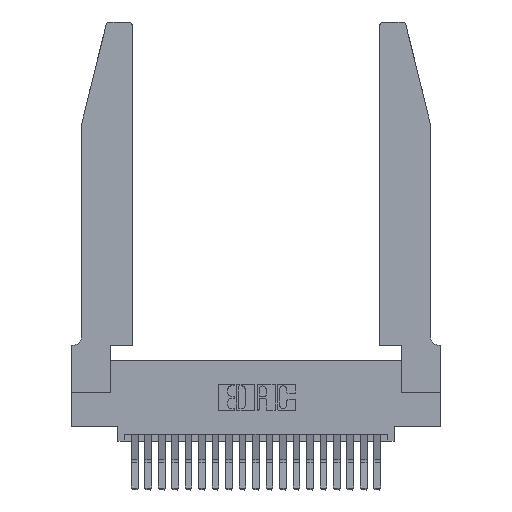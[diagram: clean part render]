
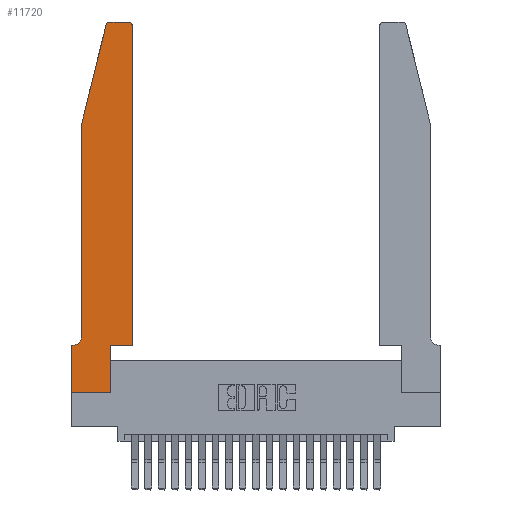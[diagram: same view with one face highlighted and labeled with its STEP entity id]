
A CAD part, top view. The second image highlights one B-rep face of the part: STEP entity #11720.
In plain terms, the highlighted planar face has unit normal (0, 0, 1).
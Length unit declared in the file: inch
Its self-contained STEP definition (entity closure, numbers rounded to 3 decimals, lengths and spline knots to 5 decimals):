
#58 = EDGE_CURVE ( 'NONE', #17497, #2567, #5552, .T. ) ;
#1557 = VECTOR ( 'NONE', #11634, 39.37008 ) ;
#1785 = CARTESIAN_POINT ( 'NONE',  ( 0.284, 2.72, 0.37 ) ) ;
#2291 = ORIENTED_EDGE ( 'NONE', *, *, #8725, .T. ) ;
#2340 = DIRECTION ( 'NONE',  ( 0., -1., 0. ) ) ;
#2380 = CARTESIAN_POINT ( 'NONE',  ( 0.0755, 0.35, 0.37 ) ) ;
#2567 = VERTEX_POINT ( 'NONE', #13069 ) ;
#2730 = VECTOR ( 'NONE', #4189, 39.37008 ) ;
#2981 = VECTOR ( 'NONE', #12494, 39.37008 ) ;
#3299 = ORIENTED_EDGE ( 'NONE', *, *, #21395, .T. ) ;
#3468 = CARTESIAN_POINT ( 'NONE',  ( 0., 0., 0.37 ) ) ;
#3584 = DIRECTION ( 'NONE',  ( 1., 0., 0. ) ) ;
#4167 = CARTESIAN_POINT ( 'NONE',  ( 0.0755, 2., 0.37 ) ) ;
#4189 = DIRECTION ( 'NONE',  ( -1., 0., 0. ) ) ;
#4584 = ORIENTED_EDGE ( 'NONE', *, *, #20979, .T. ) ;
#4935 = ORIENTED_EDGE ( 'NONE', *, *, #19337, .T. ) ;
#5075 = VERTEX_POINT ( 'NONE', #19830 ) ;
#5257 = CARTESIAN_POINT ( 'NONE',  ( 0.2865, 0., 0.37 ) ) ;
#5339 = VERTEX_POINT ( 'NONE', #6552 ) ;
#5552 = LINE ( 'NONE', #21152, #9830 ) ;
#5629 = CARTESIAN_POINT ( 'NONE',  ( 0., 0., 0.37 ) ) ;
#5875 = ORIENTED_EDGE ( 'NONE', *, *, #17522, .T. ) ;
#6082 = DIRECTION ( 'NONE',  ( 0., 0., -1. ) ) ;
#6132 = ORIENTED_EDGE ( 'NONE', *, *, #7724, .T. ) ;
#6315 = DIRECTION ( 'NONE',  ( -1., 0., 0. ) ) ;
#6552 = CARTESIAN_POINT ( 'NONE',  ( 0.4205, 2.75, 0.37 ) ) ;
#6965 = VERTEX_POINT ( 'NONE', #11075 ) ;
#7152 = DIRECTION ( 'NONE',  ( 0., 0., 1. ) ) ;
#7724 = EDGE_CURVE ( 'NONE', #5075, #22761, #13588, .T. ) ;
#8382 = CARTESIAN_POINT ( 'NONE',  ( 0.284, 2.75, 0.37 ) ) ;
#8436 = CARTESIAN_POINT ( 'NONE',  ( 0.4505, 0.35, 0.37 ) ) ;
#8725 = EDGE_CURVE ( 'NONE', #19949, #5339, #14077, .T. ) ;
#8833 = VECTOR ( 'NONE', #2340, 39.37008 ) ;
#8927 = LINE ( 'NONE', #15577, #14209 ) ;
#9027 = CARTESIAN_POINT ( 'NONE',  ( 0.0055, 0.35, 0.37 ) ) ;
#9386 = VECTOR ( 'NONE', #10244, 39.37008 ) ;
#9554 = CARTESIAN_POINT ( 'NONE',  ( 0.0755, 2., 0.37 ) ) ;
#9830 = VECTOR ( 'NONE', #10732, 39.37008 ) ;
#10030 = ORIENTED_EDGE ( 'NONE', *, *, #19240, .T. ) ;
#10244 = DIRECTION ( 'NONE',  ( 0., 1., 0. ) ) ;
#10634 = AXIS2_PLACEMENT_3D ( 'NONE', #16817, #6082, #18562 ) ;
#10695 = CIRCLE ( 'NONE', #16683, 0.03 ) ;
#10732 = DIRECTION ( 'NONE',  ( 0., 1., 0. ) ) ;
#11075 = CARTESIAN_POINT ( 'NONE',  ( 0.4505, 0.35, 0.37 ) ) ;
#11154 = VERTEX_POINT ( 'NONE', #5629 ) ;
#11178 = LINE ( 'NONE', #16906, #1557 ) ;
#11228 = DIRECTION ( 'NONE',  ( 1., 0., 0. ) ) ;
#11344 = EDGE_LOOP ( 'NONE', ( #19881, #5875, #3299, #6132, #4584, #16481, #21913, #4935, #15872, #10030, #12206, #2291 ) ) ;
#11634 = DIRECTION ( 'NONE',  ( 1., 0., 0. ) ) ;
#11720 = ADVANCED_FACE ( 'NONE', ( #22411 ), #16497, .T. ) ;
#12206 = ORIENTED_EDGE ( 'NONE', *, *, #22265, .T. ) ;
#12328 = LINE ( 'NONE', #2380, #2730 ) ;
#12494 = DIRECTION ( 'NONE',  ( 0., -1., 0. ) ) ;
#12583 = LINE ( 'NONE', #3468, #2981 ) ;
#12665 = LINE ( 'NONE', #20442, #16833 ) ;
#13056 = VECTOR ( 'NONE', #21952, 39.37008 ) ;
#13069 = CARTESIAN_POINT ( 'NONE',  ( 0.2865, 0.35, 0.37 ) ) ;
#13264 = CARTESIAN_POINT ( 'NONE',  ( 0.25487, 2.72718, 0.37 ) ) ;
#13588 = LINE ( 'NONE', #9554, #8833 ) ;
#14077 = CIRCLE ( 'NONE', #21797, 0.03 ) ;
#14111 = LINE ( 'NONE', #8436, #9386 ) ;
#14209 = VECTOR ( 'NONE', #17148, 39.37008 ) ;
#14366 = DIRECTION ( 'NONE',  ( 0., 0., 1. ) ) ;
#14715 = CARTESIAN_POINT ( 'NONE',  ( 0., 0.35, 0.37 ) ) ;
#15268 = CARTESIAN_POINT ( 'NONE',  ( 0.0755, 0.42, 0.37 ) ) ;
#15559 = AXIS2_PLACEMENT_3D ( 'NONE', #14715, #21748, #11228 ) ;
#15577 = CARTESIAN_POINT ( 'NONE',  ( 0., 0., 0.37 ) ) ;
#15872 = ORIENTED_EDGE ( 'NONE', *, *, #58, .T. ) ;
#16481 = ORIENTED_EDGE ( 'NONE', *, *, #18370, .T. ) ;
#16497 = PLANE ( 'NONE',  #15559 ) ;
#16677 = CIRCLE ( 'NONE', #10634, 0.07 ) ;
#16683 = AXIS2_PLACEMENT_3D ( 'NONE', #1785, #14366, #3584 ) ;
#16817 = CARTESIAN_POINT ( 'NONE',  ( 0.0055, 0.42, 0.37 ) ) ;
#16833 = VECTOR ( 'NONE', #6315, 39.37008 ) ;
#16885 = VERTEX_POINT ( 'NONE', #9027 ) ;
#16906 = CARTESIAN_POINT ( 'NONE',  ( 0.4505, 0.35, 0.37 ) ) ;
#17148 = DIRECTION ( 'NONE',  ( 1., 0., 0. ) ) ;
#17203 = EDGE_CURVE ( 'NONE', #5339, #21588, #12665, .T. ) ;
#17497 = VERTEX_POINT ( 'NONE', #5257 ) ;
#17522 = EDGE_CURVE ( 'NONE', #21588, #19210, #10695, .T. ) ;
#17816 = CARTESIAN_POINT ( 'NONE',  ( 0.4205, 2.72, 0.37 ) ) ;
#18370 = EDGE_CURVE ( 'NONE', #16885, #21898, #12328, .T. ) ;
#18562 = DIRECTION ( 'NONE',  ( -1., 0., 0. ) ) ;
#18920 = CARTESIAN_POINT ( 'NONE',  ( 0.4505, 2.72, 0.37 ) ) ;
#18947 = EDGE_CURVE ( 'NONE', #21898, #11154, #12583, .T. ) ;
#19210 = VERTEX_POINT ( 'NONE', #13264 ) ;
#19240 = EDGE_CURVE ( 'NONE', #2567, #6965, #11178, .T. ) ;
#19337 = EDGE_CURVE ( 'NONE', #11154, #17497, #8927, .T. ) ;
#19569 = DIRECTION ( 'NONE',  ( 1., 0., 0. ) ) ;
#19830 = CARTESIAN_POINT ( 'NONE',  ( 0.0755, 2., 0.37 ) ) ;
#19881 = ORIENTED_EDGE ( 'NONE', *, *, #17203, .T. ) ;
#19949 = VERTEX_POINT ( 'NONE', #18920 ) ;
#20442 = CARTESIAN_POINT ( 'NONE',  ( 0.2605, 2.75, 0.37 ) ) ;
#20979 = EDGE_CURVE ( 'NONE', #22761, #16885, #16677, .T. ) ;
#21152 = CARTESIAN_POINT ( 'NONE',  ( 0.2865, 0.35, 0.37 ) ) ;
#21395 = EDGE_CURVE ( 'NONE', #19210, #5075, #22339, .T. ) ;
#21491 = CARTESIAN_POINT ( 'NONE',  ( 0., 0.35, 0.37 ) ) ;
#21588 = VERTEX_POINT ( 'NONE', #8382 ) ;
#21748 = DIRECTION ( 'NONE',  ( 0., 0., 1. ) ) ;
#21797 = AXIS2_PLACEMENT_3D ( 'NONE', #17816, #7152, #19569 ) ;
#21898 = VERTEX_POINT ( 'NONE', #21491 ) ;
#21913 = ORIENTED_EDGE ( 'NONE', *, *, #18947, .T. ) ;
#21952 = DIRECTION ( 'NONE',  ( -0.239, -0.971, 0. ) ) ;
#22265 = EDGE_CURVE ( 'NONE', #6965, #19949, #14111, .T. ) ;
#22339 = LINE ( 'NONE', #4167, #13056 ) ;
#22411 = FACE_OUTER_BOUND ( 'NONE', #11344, .T. ) ;
#22761 = VERTEX_POINT ( 'NONE', #15268 ) ;
